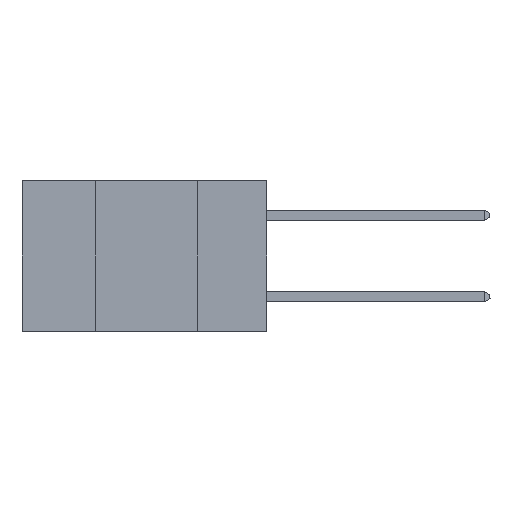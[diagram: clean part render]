
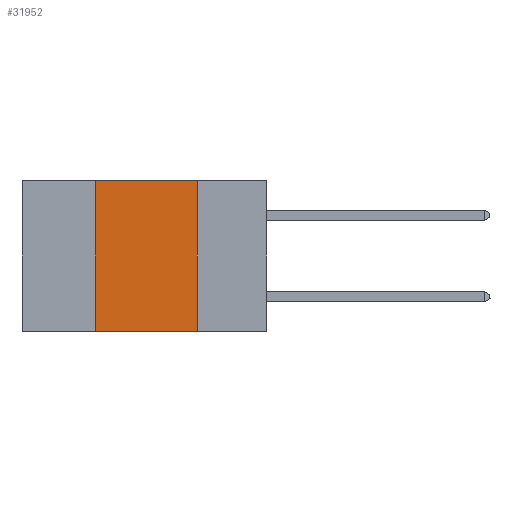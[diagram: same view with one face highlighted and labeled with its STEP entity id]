
A CAD part, left-side view. The second image highlights one B-rep face of the part: STEP entity #31952.
In plain terms, the highlighted planar face has unit normal (-1, 0, 0).
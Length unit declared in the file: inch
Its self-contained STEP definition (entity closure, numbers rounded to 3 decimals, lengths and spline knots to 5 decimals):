
#265 = VECTOR ( 'NONE', #33478, 39.37008 ) ;
#310 = LINE ( 'NONE', #4727, #265 ) ;
#3504 = CARTESIAN_POINT ( 'NONE',  ( 0., 0.17, 0. ) ) ;
#3534 = CARTESIAN_POINT ( 'NONE',  ( 0., 0.42, 0. ) ) ;
#3881 = FACE_OUTER_BOUND ( 'NONE', #17106, .T. ) ;
#4278 = EDGE_CURVE ( 'NONE', #23151, #17513, #310, .T. ) ;
#4727 = CARTESIAN_POINT ( 'NONE',  ( 0., 0.42, 0. ) ) ;
#4806 = AXIS2_PLACEMENT_3D ( 'NONE', #22728, #11983, #36521 ) ;
#6908 = CARTESIAN_POINT ( 'NONE',  ( 0., 0.17, -0.37 ) ) ;
#8283 = PLANE ( 'NONE',  #4806 ) ;
#11408 = ORIENTED_EDGE ( 'NONE', *, *, #36223, .F. ) ;
#11983 = DIRECTION ( 'NONE',  ( 1., 0., 0. ) ) ;
#12342 = LINE ( 'NONE', #3504, #39069 ) ;
#13194 = DIRECTION ( 'NONE',  ( 0., -1., 0. ) ) ;
#14919 = CARTESIAN_POINT ( 'NONE',  ( 0., 0.42, -0.37 ) ) ;
#16548 = CARTESIAN_POINT ( 'NONE',  ( 0., 0.17, 0. ) ) ;
#17106 = EDGE_LOOP ( 'NONE', ( #11408, #20972, #20000, #25125 ) ) ;
#17513 = VERTEX_POINT ( 'NONE', #3534 ) ;
#19166 = VERTEX_POINT ( 'NONE', #6908 ) ;
#20000 = ORIENTED_EDGE ( 'NONE', *, *, #4278, .F. ) ;
#20472 = LINE ( 'NONE', #44225, #30800 ) ;
#20931 = EDGE_CURVE ( 'NONE', #23151, #19166, #20472, .T. ) ;
#20972 = ORIENTED_EDGE ( 'NONE', *, *, #31252, .F. ) ;
#22728 = CARTESIAN_POINT ( 'NONE',  ( 0., 0.6, 0. ) ) ;
#23151 = VERTEX_POINT ( 'NONE', #14919 ) ;
#25125 = ORIENTED_EDGE ( 'NONE', *, *, #20931, .T. ) ;
#26245 = VECTOR ( 'NONE', #39471, 39.37008 ) ;
#27347 = LINE ( 'NONE', #42789, #26245 ) ;
#28902 = DIRECTION ( 'NONE',  ( 0., 0., -1. ) ) ;
#30800 = VECTOR ( 'NONE', #13194, 39.37008 ) ;
#31252 = EDGE_CURVE ( 'NONE', #17513, #41984, #27347, .T. ) ;
#31952 = ADVANCED_FACE ( 'NONE', ( #3881 ), #8283, .F. ) ;
#33478 = DIRECTION ( 'NONE',  ( 0., 0., 1. ) ) ;
#36223 = EDGE_CURVE ( 'NONE', #41984, #19166, #12342, .T. ) ;
#36521 = DIRECTION ( 'NONE',  ( 0., 0., -1. ) ) ;
#39069 = VECTOR ( 'NONE', #28902, 39.37008 ) ;
#39471 = DIRECTION ( 'NONE',  ( 0., -1., 0. ) ) ;
#41984 = VERTEX_POINT ( 'NONE', #16548 ) ;
#42789 = CARTESIAN_POINT ( 'NONE',  ( 0., 0.6, 0. ) ) ;
#44225 = CARTESIAN_POINT ( 'NONE',  ( 0., 0.6, -0.37 ) ) ;
